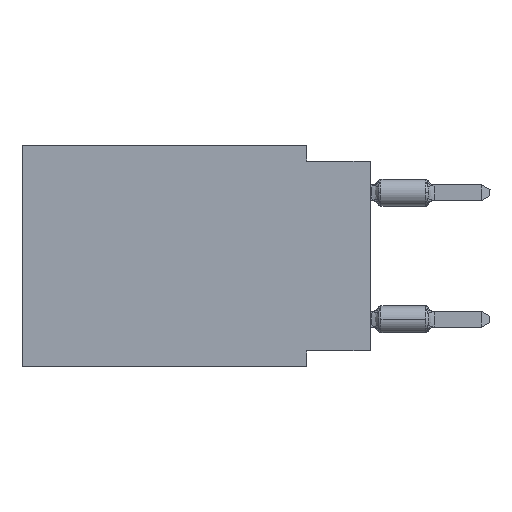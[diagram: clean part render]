
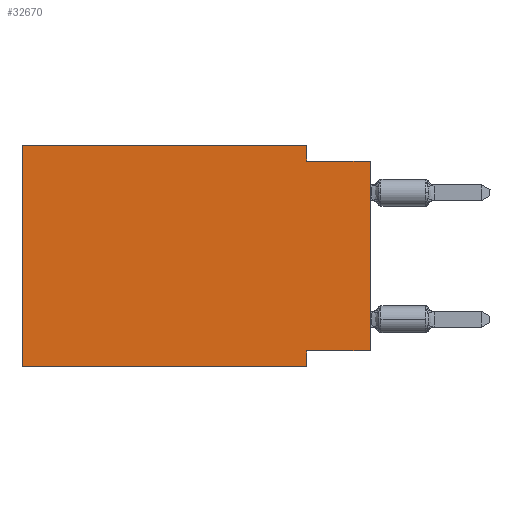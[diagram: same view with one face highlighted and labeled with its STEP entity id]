
A CAD part, left-side view. The second image highlights one B-rep face of the part: STEP entity #32670.
In plain terms, the highlighted planar face has unit normal (-1, 0, 0).
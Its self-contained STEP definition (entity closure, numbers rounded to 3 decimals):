
#1244 = LINE ( 'NONE', #4000, #19976 ) ;
#1951 = FACE_OUTER_BOUND ( 'NONE', #4151, .T. ) ;
#2020 = CARTESIAN_POINT ( 'NONE',  ( 0., 0., -0.635 ) ) ;
#2477 = CARTESIAN_POINT ( 'NONE',  ( 0., 13.97, 0. ) ) ;
#3236 = LINE ( 'NONE', #18980, #6231 ) ;
#3618 = CARTESIAN_POINT ( 'NONE',  ( 0., 2.54, -8.255 ) ) ;
#4000 = CARTESIAN_POINT ( 'NONE',  ( 0., 0., 0. ) ) ;
#4002 = CARTESIAN_POINT ( 'NONE',  ( 0., 13.97, 0. ) ) ;
#4151 = EDGE_LOOP ( 'NONE', ( #21331, #35975, #22952, #4279, #34107, #14379, #31210, #29026 ) ) ;
#4279 = ORIENTED_EDGE ( 'NONE', *, *, #35834, .F. ) ;
#4353 = AXIS2_PLACEMENT_3D ( 'NONE', #11587, #14349, #37736 ) ;
#5280 = PLANE ( 'NONE',  #4353 ) ;
#6231 = VECTOR ( 'NONE', #18399, 1000. ) ;
#6820 = EDGE_CURVE ( 'NONE', #33100, #28393, #35981, .T. ) ;
#7824 = VERTEX_POINT ( 'NONE', #32065 ) ;
#7849 = LINE ( 'NONE', #38091, #36878 ) ;
#8663 = DIRECTION ( 'NONE',  ( 0., 0., -1. ) ) ;
#9598 = VECTOR ( 'NONE', #22299, 1000. ) ;
#9886 = CARTESIAN_POINT ( 'NONE',  ( 0., 13.97, 0. ) ) ;
#10011 = CARTESIAN_POINT ( 'NONE',  ( 0., 13.97, -8.89 ) ) ;
#11566 = VERTEX_POINT ( 'NONE', #21503 ) ;
#11587 = CARTESIAN_POINT ( 'NONE',  ( 0., 13.97, 0. ) ) ;
#11596 = EDGE_CURVE ( 'NONE', #11566, #7824, #1244, .T. ) ;
#14349 = DIRECTION ( 'NONE',  ( 1., 0., 0. ) ) ;
#14379 = ORIENTED_EDGE ( 'NONE', *, *, #29199, .T. ) ;
#17131 = EDGE_CURVE ( 'NONE', #29956, #23212, #23955, .T. ) ;
#17172 = DIRECTION ( 'NONE',  ( 0., -1., 0. ) ) ;
#18399 = DIRECTION ( 'NONE',  ( 0., 1., 0. ) ) ;
#18980 = CARTESIAN_POINT ( 'NONE',  ( 0., 0., -8.255 ) ) ;
#19373 = VERTEX_POINT ( 'NONE', #2477 ) ;
#19976 = VECTOR ( 'NONE', #21697, 1000. ) ;
#21331 = ORIENTED_EDGE ( 'NONE', *, *, #11596, .T. ) ;
#21428 = CARTESIAN_POINT ( 'NONE',  ( 0., 2.54, 0. ) ) ;
#21503 = CARTESIAN_POINT ( 'NONE',  ( 0., 0., -8.255 ) ) ;
#21697 = DIRECTION ( 'NONE',  ( 0., 0., 1. ) ) ;
#21850 = VECTOR ( 'NONE', #35540, 1000. ) ;
#22096 = LINE ( 'NONE', #4002, #9598 ) ;
#22299 = DIRECTION ( 'NONE',  ( 0., 0., 1. ) ) ;
#22556 = CARTESIAN_POINT ( 'NONE',  ( 0., 2.54, -0.635 ) ) ;
#22607 = DIRECTION ( 'NONE',  ( 0., -1., 0. ) ) ;
#22952 = ORIENTED_EDGE ( 'NONE', *, *, #6820, .F. ) ;
#23212 = VERTEX_POINT ( 'NONE', #29365 ) ;
#23955 = LINE ( 'NONE', #38105, #21850 ) ;
#25671 = EDGE_CURVE ( 'NONE', #28393, #7824, #26393, .T. ) ;
#26393 = LINE ( 'NONE', #2020, #35804 ) ;
#28393 = VERTEX_POINT ( 'NONE', #22556 ) ;
#29026 = ORIENTED_EDGE ( 'NONE', *, *, #31131, .F. ) ;
#29199 = EDGE_CURVE ( 'NONE', #37996, #23212, #7849, .T. ) ;
#29365 = CARTESIAN_POINT ( 'NONE',  ( 0., 2.54, -8.89 ) ) ;
#29956 = VERTEX_POINT ( 'NONE', #3618 ) ;
#31131 = EDGE_CURVE ( 'NONE', #11566, #29956, #3236, .T. ) ;
#31210 = ORIENTED_EDGE ( 'NONE', *, *, #17131, .F. ) ;
#31986 = CARTESIAN_POINT ( 'NONE',  ( 0., 2.54, 0. ) ) ;
#32065 = CARTESIAN_POINT ( 'NONE',  ( 0., 0., -0.635 ) ) ;
#32670 = ADVANCED_FACE ( 'NONE', ( #1951 ), #5280, .F. ) ;
#33076 = LINE ( 'NONE', #9886, #38476 ) ;
#33100 = VERTEX_POINT ( 'NONE', #31986 ) ;
#34107 = ORIENTED_EDGE ( 'NONE', *, *, #34987, .F. ) ;
#34443 = VECTOR ( 'NONE', #8663, 1000. ) ;
#34987 = EDGE_CURVE ( 'NONE', #37996, #19373, #22096, .T. ) ;
#35540 = DIRECTION ( 'NONE',  ( 0., 0., -1. ) ) ;
#35804 = VECTOR ( 'NONE', #17172, 1000. ) ;
#35834 = EDGE_CURVE ( 'NONE', #19373, #33100, #33076, .T. ) ;
#35975 = ORIENTED_EDGE ( 'NONE', *, *, #25671, .F. ) ;
#35981 = LINE ( 'NONE', #21428, #34443 ) ;
#36222 = DIRECTION ( 'NONE',  ( 0., -1., 0. ) ) ;
#36878 = VECTOR ( 'NONE', #22607, 1000. ) ;
#37736 = DIRECTION ( 'NONE',  ( 0., 0., -1. ) ) ;
#37996 = VERTEX_POINT ( 'NONE', #10011 ) ;
#38091 = CARTESIAN_POINT ( 'NONE',  ( 0., 13.97, -8.89 ) ) ;
#38105 = CARTESIAN_POINT ( 'NONE',  ( 0., 2.54, -8.89 ) ) ;
#38476 = VECTOR ( 'NONE', #36222, 1000. ) ;
